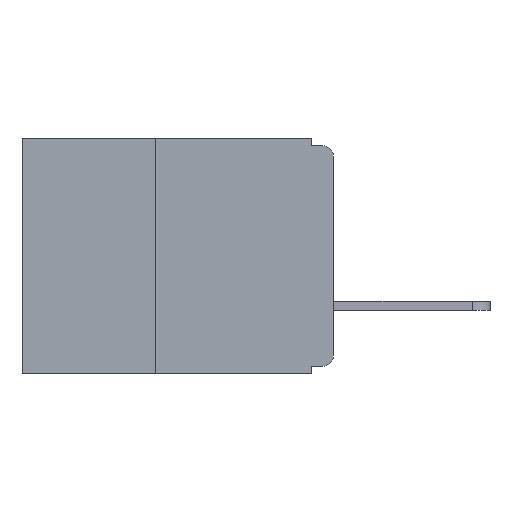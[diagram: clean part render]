
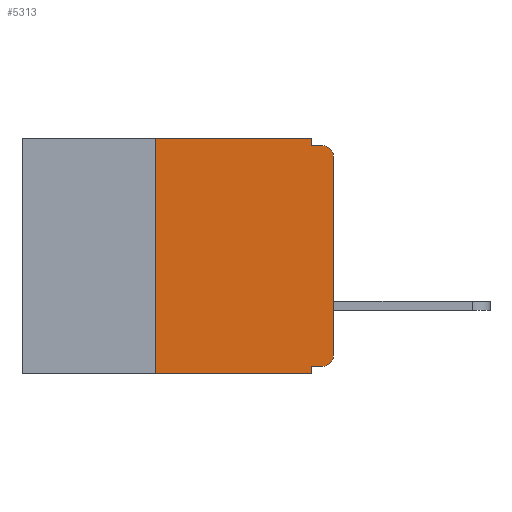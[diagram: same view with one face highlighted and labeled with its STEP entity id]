
A CAD part, left-side view. The second image highlights one B-rep face of the part: STEP entity #5313.
In plain terms, the highlighted planar face has unit normal (-1, 0, 0).
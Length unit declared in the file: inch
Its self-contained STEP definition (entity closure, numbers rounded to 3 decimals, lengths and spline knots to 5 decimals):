
#26 = ORIENTED_EDGE ( 'NONE', *, *, #5025, .T. ) ;
#131 = FACE_OUTER_BOUND ( 'NONE', #1004, .T. ) ;
#603 = CARTESIAN_POINT ( 'NONE',  ( 0., 0., -0.305 ) ) ;
#608 = DIRECTION ( 'NONE',  ( 0., 0., -1. ) ) ;
#1004 = EDGE_LOOP ( 'NONE', ( #4755, #26, #3689, #9818, #12035, #2495, #14696, #14504, #12114, #3550 ) ) ;
#1041 = CIRCLE ( 'NONE', #10003, 0.015 ) ;
#1279 = LINE ( 'NONE', #6232, #9492 ) ;
#1293 = VERTEX_POINT ( 'NONE', #603 ) ;
#1427 = VECTOR ( 'NONE', #9396, 39.37008 ) ;
#1843 = EDGE_CURVE ( 'NONE', #14056, #6581, #7694, .T. ) ;
#1862 = EDGE_CURVE ( 'NONE', #6028, #14056, #4243, .T. ) ;
#2311 = DIRECTION ( 'NONE',  ( 0., -1., 0. ) ) ;
#2433 = DIRECTION ( 'NONE',  ( 0., -1., 0. ) ) ;
#2495 = ORIENTED_EDGE ( 'NONE', *, *, #1862, .F. ) ;
#2534 = CARTESIAN_POINT ( 'NONE',  ( 0., 0.015, -0.025 ) ) ;
#2650 = VERTEX_POINT ( 'NONE', #10563 ) ;
#2719 = CARTESIAN_POINT ( 'NONE',  ( 0., 0.25, -0.33 ) ) ;
#2885 = AXIS2_PLACEMENT_3D ( 'NONE', #7053, #9612, #6547 ) ;
#3030 = CARTESIAN_POINT ( 'NONE',  ( 0., 0.031, -0.33 ) ) ;
#3089 = EDGE_CURVE ( 'NONE', #14405, #10686, #9489, .T. ) ;
#3159 = VECTOR ( 'NONE', #2433, 39.37008 ) ;
#3202 = VERTEX_POINT ( 'NONE', #13092 ) ;
#3496 = CARTESIAN_POINT ( 'NONE',  ( 0., 0.015, -0.01 ) ) ;
#3550 = ORIENTED_EDGE ( 'NONE', *, *, #5932, .T. ) ;
#3689 = ORIENTED_EDGE ( 'NONE', *, *, #3089, .F. ) ;
#3690 = CARTESIAN_POINT ( 'NONE',  ( 0., 0.25, -0.33 ) ) ;
#3752 = CARTESIAN_POINT ( 'NONE',  ( 0., 0.031, 0. ) ) ;
#3932 = VECTOR ( 'NONE', #4851, 39.37008 ) ;
#4243 = LINE ( 'NONE', #3690, #14294 ) ;
#4755 = ORIENTED_EDGE ( 'NONE', *, *, #8674, .T. ) ;
#4796 = CARTESIAN_POINT ( 'NONE',  ( 0., 0.437, -0.33 ) ) ;
#4851 = DIRECTION ( 'NONE',  ( 0., -1., 0. ) ) ;
#5025 = EDGE_CURVE ( 'NONE', #3202, #10686, #1041, .T. ) ;
#5313 = ADVANCED_FACE ( 'NONE', ( #131 ), #9532, .F. ) ;
#5392 = CIRCLE ( 'NONE', #14018, 0.015 ) ;
#5598 = EDGE_CURVE ( 'NONE', #6028, #12936, #11039, .T. ) ;
#5932 = EDGE_CURVE ( 'NONE', #2650, #1293, #5392, .T. ) ;
#5971 = DIRECTION ( 'NONE',  ( 0., 0., 1. ) ) ;
#6028 = VERTEX_POINT ( 'NONE', #2719 ) ;
#6232 = CARTESIAN_POINT ( 'NONE',  ( 0., 0.031, -0.33 ) ) ;
#6378 = DIRECTION ( 'NONE',  ( 0., 1., 0. ) ) ;
#6481 = CARTESIAN_POINT ( 'NONE',  ( 0., 0., -0.32 ) ) ;
#6511 = DIRECTION ( 'NONE',  ( 0., 0., 1. ) ) ;
#6547 = DIRECTION ( 'NONE',  ( 0., 0., -1. ) ) ;
#6581 = VERTEX_POINT ( 'NONE', #3752 ) ;
#7026 = CARTESIAN_POINT ( 'NONE',  ( 0., 0.031, -0.01 ) ) ;
#7053 = CARTESIAN_POINT ( 'NONE',  ( 0., 0.437, 0. ) ) ;
#7292 = VECTOR ( 'NONE', #6378, 39.37008 ) ;
#7594 = CARTESIAN_POINT ( 'NONE',  ( 0., 0.031, -0.32 ) ) ;
#7694 = LINE ( 'NONE', #14155, #3159 ) ;
#7984 = EDGE_CURVE ( 'NONE', #2650, #14008, #13738, .T. ) ;
#8605 = CARTESIAN_POINT ( 'NONE',  ( 0., 0.015, -0.305 ) ) ;
#8674 = EDGE_CURVE ( 'NONE', #1293, #3202, #13893, .T. ) ;
#8744 = CARTESIAN_POINT ( 'NONE',  ( 0., 0., 0. ) ) ;
#9396 = DIRECTION ( 'NONE',  ( 0., 0., -1. ) ) ;
#9489 = LINE ( 'NONE', #10294, #12599 ) ;
#9492 = VECTOR ( 'NONE', #12026, 39.37008 ) ;
#9532 = PLANE ( 'NONE',  #2885 ) ;
#9612 = DIRECTION ( 'NONE',  ( 1., 0., 0. ) ) ;
#9762 = EDGE_CURVE ( 'NONE', #6581, #14405, #11830, .T. ) ;
#9818 = ORIENTED_EDGE ( 'NONE', *, *, #9762, .F. ) ;
#9945 = DIRECTION ( 'NONE',  ( -1., 0., 0. ) ) ;
#10003 = AXIS2_PLACEMENT_3D ( 'NONE', #2534, #10674, #11854 ) ;
#10294 = CARTESIAN_POINT ( 'NONE',  ( 0., 0., -0.01 ) ) ;
#10563 = CARTESIAN_POINT ( 'NONE',  ( 0., 0.015, -0.32 ) ) ;
#10674 = DIRECTION ( 'NONE',  ( -1., 0., 0. ) ) ;
#10686 = VERTEX_POINT ( 'NONE', #3496 ) ;
#11030 = CARTESIAN_POINT ( 'NONE',  ( 0., 0.25, 0. ) ) ;
#11039 = LINE ( 'NONE', #4796, #3932 ) ;
#11830 = LINE ( 'NONE', #14026, #1427 ) ;
#11854 = DIRECTION ( 'NONE',  ( 0., 0., -1. ) ) ;
#12026 = DIRECTION ( 'NONE',  ( 0., 0., -1. ) ) ;
#12035 = ORIENTED_EDGE ( 'NONE', *, *, #1843, .F. ) ;
#12058 = VECTOR ( 'NONE', #6511, 39.37008 ) ;
#12114 = ORIENTED_EDGE ( 'NONE', *, *, #7984, .F. ) ;
#12599 = VECTOR ( 'NONE', #2311, 39.37008 ) ;
#12936 = VERTEX_POINT ( 'NONE', #3030 ) ;
#13092 = CARTESIAN_POINT ( 'NONE',  ( 0., 0., -0.025 ) ) ;
#13474 = EDGE_CURVE ( 'NONE', #14008, #12936, #1279, .T. ) ;
#13738 = LINE ( 'NONE', #6481, #7292 ) ;
#13893 = LINE ( 'NONE', #8744, #12058 ) ;
#14008 = VERTEX_POINT ( 'NONE', #7594 ) ;
#14018 = AXIS2_PLACEMENT_3D ( 'NONE', #8605, #9945, #608 ) ;
#14026 = CARTESIAN_POINT ( 'NONE',  ( 0., 0.031, 0. ) ) ;
#14056 = VERTEX_POINT ( 'NONE', #11030 ) ;
#14155 = CARTESIAN_POINT ( 'NONE',  ( 0., 0.437, 0. ) ) ;
#14294 = VECTOR ( 'NONE', #5971, 39.37008 ) ;
#14405 = VERTEX_POINT ( 'NONE', #7026 ) ;
#14504 = ORIENTED_EDGE ( 'NONE', *, *, #13474, .F. ) ;
#14696 = ORIENTED_EDGE ( 'NONE', *, *, #5598, .T. ) ;
